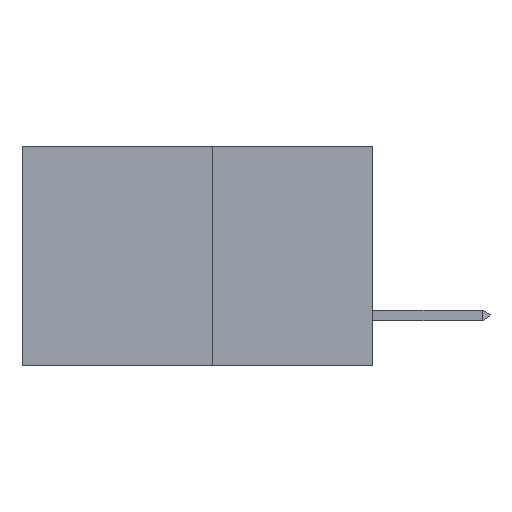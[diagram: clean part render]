
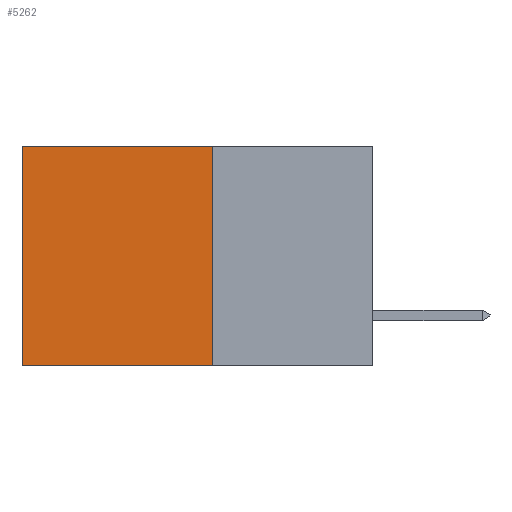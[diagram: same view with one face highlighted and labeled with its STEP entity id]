
A CAD part, left-side view. The second image highlights one B-rep face of the part: STEP entity #5262.
In plain terms, the highlighted planar face has unit normal (-1, 0, 0).
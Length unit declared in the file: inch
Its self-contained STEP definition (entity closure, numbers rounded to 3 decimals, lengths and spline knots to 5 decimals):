
#2983 = CARTESIAN_POINT ( 'NONE',  ( 0.277, 0.27, -0.37 ) ) ;
#4133 = DIRECTION ( 'NONE',  ( 0., 0., -1. ) ) ;
#4139 = DIRECTION ( 'NONE',  ( 1., 0., 0. ) ) ;
#4214 = CARTESIAN_POINT ( 'NONE',  ( 0.277, 0.27, -0.37 ) ) ;
#4338 = DIRECTION ( 'NONE',  ( 0., 0., -1. ) ) ;
#4381 = PLANE ( 'NONE',  #7274 ) ;
#4511 = CARTESIAN_POINT ( 'NONE',  ( 0.277, 0.27, 0. ) ) ;
#4868 = CARTESIAN_POINT ( 'NONE',  ( 0.277, 0.27, -0.37 ) ) ;
#5262 = ADVANCED_FACE ( 'NONE', ( #5338 ), #4381, .F. ) ;
#5338 = FACE_OUTER_BOUND ( 'NONE', #24286, .T. ) ;
#5437 = VECTOR ( 'NONE', #9592, 39.37008 ) ;
#5986 = CARTESIAN_POINT ( 'NONE',  ( 0.277, 0.59, 0. ) ) ;
#7274 = AXIS2_PLACEMENT_3D ( 'NONE', #4214, #4139, #4133 ) ;
#7400 = DIRECTION ( 'NONE',  ( 0., 0., -1. ) ) ;
#9491 = CARTESIAN_POINT ( 'NONE',  ( 0.277, 0.27, 0. ) ) ;
#9492 = VERTEX_POINT ( 'NONE', #9491 ) ;
#9592 = DIRECTION ( 'NONE',  ( 0., 1., 0. ) ) ;
#12209 = ORIENTED_EDGE ( 'NONE', *, *, #25631, .F. ) ;
#15631 = LINE ( 'NONE', #18884, #28947 ) ;
#16249 = VECTOR ( 'NONE', #7400, 39.37008 ) ;
#16908 = CARTESIAN_POINT ( 'NONE',  ( 0.277, 0.59, -0.37 ) ) ;
#18755 = ORIENTED_EDGE ( 'NONE', *, *, #28672, .T. ) ;
#18884 = CARTESIAN_POINT ( 'NONE',  ( 0.277, 0.27, -0.37 ) ) ;
#19003 = CARTESIAN_POINT ( 'NONE',  ( 0.277, 0.59, -0.37 ) ) ;
#20581 = VERTEX_POINT ( 'NONE', #5986 ) ;
#20939 = EDGE_CURVE ( 'NONE', #9492, #21120, #29567, .T. ) ;
#21120 = VERTEX_POINT ( 'NONE', #2983 ) ;
#24075 = EDGE_CURVE ( 'NONE', #9492, #20581, #32163, .T. ) ;
#24286 = EDGE_LOOP ( 'NONE', ( #18755, #12209, #29701, #24889 ) ) ;
#24831 = VECTOR ( 'NONE', #4338, 39.37008 ) ;
#24889 = ORIENTED_EDGE ( 'NONE', *, *, #24075, .T. ) ;
#25631 = EDGE_CURVE ( 'NONE', #21120, #25650, #15631, .T. ) ;
#25650 = VERTEX_POINT ( 'NONE', #19003 ) ;
#26300 = DIRECTION ( 'NONE',  ( 0., 1., 0. ) ) ;
#28672 = EDGE_CURVE ( 'NONE', #20581, #25650, #32267, .T. ) ;
#28947 = VECTOR ( 'NONE', #26300, 39.37008 ) ;
#29567 = LINE ( 'NONE', #4868, #16249 ) ;
#29701 = ORIENTED_EDGE ( 'NONE', *, *, #20939, .F. ) ;
#32163 = LINE ( 'NONE', #4511, #5437 ) ;
#32267 = LINE ( 'NONE', #16908, #24831 ) ;
